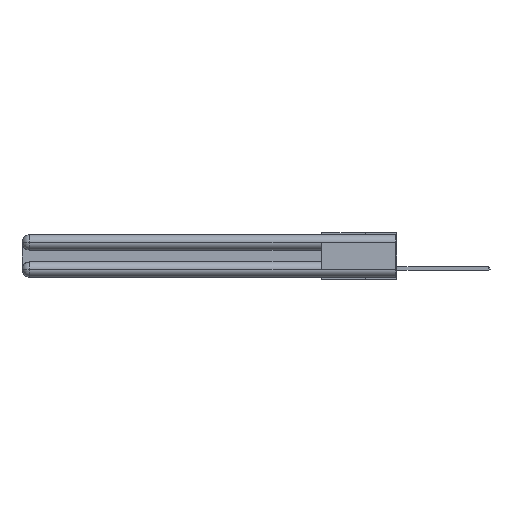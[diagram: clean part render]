
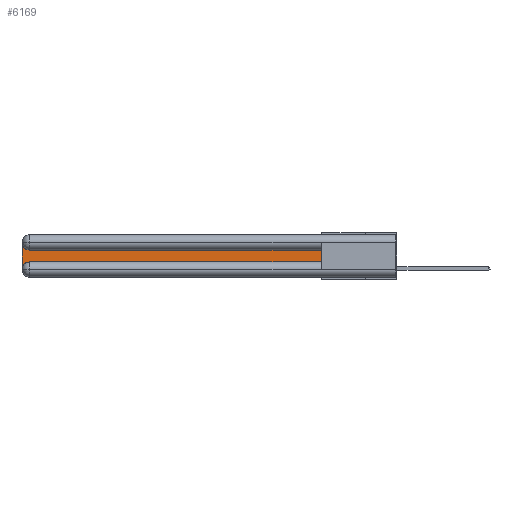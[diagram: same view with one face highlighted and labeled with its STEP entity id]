
A CAD part, left-side view. The second image highlights one B-rep face of the part: STEP entity #6169.
In plain terms, the highlighted planar face has unit normal (-1, 0, 0).
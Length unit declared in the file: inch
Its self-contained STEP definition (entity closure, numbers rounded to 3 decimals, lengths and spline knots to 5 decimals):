
#395 = DIRECTION ( 'NONE',  ( 0., -1., 0. ) ) ;
#704 = VERTEX_POINT ( 'NONE', #10089 ) ;
#2529 = ORIENTED_EDGE ( 'NONE', *, *, #26512, .T. ) ;
#2551 = CARTESIAN_POINT ( 'NONE',  ( 0.075, 2.94, -0.0625 ) ) ;
#2693 = ORIENTED_EDGE ( 'NONE', *, *, #11788, .T. ) ;
#3070 = CARTESIAN_POINT ( 'NONE',  ( 0.075, 3., -0.0625 ) ) ;
#3834 = CARTESIAN_POINT ( 'NONE',  ( 0.075, 2.94, -0.2775 ) ) ;
#5436 = ORIENTED_EDGE ( 'NONE', *, *, #26679, .T. ) ;
#5887 = DIRECTION ( 'NONE',  ( 1., 0., 0. ) ) ;
#6169 = ADVANCED_FACE ( 'NONE', ( #20670 ), #20953, .F. ) ;
#6573 = LINE ( 'NONE', #13060, #21258 ) ;
#6586 = ORIENTED_EDGE ( 'NONE', *, *, #11910, .T. ) ;
#7277 = DIRECTION ( 'NONE',  ( 0., 0., -1. ) ) ;
#7910 = CIRCLE ( 'NONE', #12786, 0.06 ) ;
#7993 = CARTESIAN_POINT ( 'NONE',  ( 0.075, 0.6, -0.2175 ) ) ;
#8329 = VERTEX_POINT ( 'NONE', #24337 ) ;
#9849 = AXIS2_PLACEMENT_3D ( 'NONE', #21363, #16585, #28804 ) ;
#10089 = CARTESIAN_POINT ( 'NONE',  ( 0.075, 0.6, -0.1225 ) ) ;
#10375 = CARTESIAN_POINT ( 'NONE',  ( 0.075, 3., -0.2775 ) ) ;
#11788 = EDGE_CURVE ( 'NONE', #22066, #704, #6573, .T. ) ;
#11910 = EDGE_CURVE ( 'NONE', #704, #8329, #26477, .T. ) ;
#12786 = AXIS2_PLACEMENT_3D ( 'NONE', #2551, #24710, #20321 ) ;
#13060 = CARTESIAN_POINT ( 'NONE',  ( 0.075, 0.6, -0.2175 ) ) ;
#14598 = VECTOR ( 'NONE', #24928, 39.37008 ) ;
#14994 = LINE ( 'NONE', #19904, #19874 ) ;
#15702 = CARTESIAN_POINT ( 'NONE',  ( 0.075, 2.94, -0.2175 ) ) ;
#16585 = DIRECTION ( 'NONE',  ( 1., 0., 0. ) ) ;
#16962 = ORIENTED_EDGE ( 'NONE', *, *, #27528, .T. ) ;
#17598 = ORIENTED_EDGE ( 'NONE', *, *, #28688, .T. ) ;
#18393 = CARTESIAN_POINT ( 'NONE',  ( 0.075, 3., -0.2175 ) ) ;
#18970 = AXIS2_PLACEMENT_3D ( 'NONE', #3834, #5887, #26029 ) ;
#19874 = VECTOR ( 'NONE', #395, 39.37008 ) ;
#19904 = CARTESIAN_POINT ( 'NONE',  ( 0.075, 0.6, -0.2175 ) ) ;
#20286 = CIRCLE ( 'NONE', #18970, 0.06 ) ;
#20321 = DIRECTION ( 'NONE',  ( 0., 0., -1. ) ) ;
#20486 = VERTEX_POINT ( 'NONE', #15702 ) ;
#20670 = FACE_OUTER_BOUND ( 'NONE', #24017, .T. ) ;
#20953 = PLANE ( 'NONE',  #9849 ) ;
#21258 = VECTOR ( 'NONE', #24358, 39.37008 ) ;
#21363 = CARTESIAN_POINT ( 'NONE',  ( 0.075, 3., -0.1225 ) ) ;
#22066 = VERTEX_POINT ( 'NONE', #7993 ) ;
#22728 = VECTOR ( 'NONE', #7277, 39.37008 ) ;
#24017 = EDGE_LOOP ( 'NONE', ( #6586, #17598, #2529, #5436, #16962, #2693 ) ) ;
#24112 = LINE ( 'NONE', #18393, #22728 ) ;
#24337 = CARTESIAN_POINT ( 'NONE',  ( 0.075, 2.94, -0.1225 ) ) ;
#24358 = DIRECTION ( 'NONE',  ( 0., 0., 1. ) ) ;
#24461 = VERTEX_POINT ( 'NONE', #3070 ) ;
#24654 = CARTESIAN_POINT ( 'NONE',  ( 0.075, 0.6, -0.1225 ) ) ;
#24675 = VERTEX_POINT ( 'NONE', #10375 ) ;
#24710 = DIRECTION ( 'NONE',  ( 1., 0., 0. ) ) ;
#24928 = DIRECTION ( 'NONE',  ( 0., 1., 0. ) ) ;
#26029 = DIRECTION ( 'NONE',  ( 0., 0., -1. ) ) ;
#26477 = LINE ( 'NONE', #24654, #14598 ) ;
#26512 = EDGE_CURVE ( 'NONE', #24461, #24675, #24112, .T. ) ;
#26679 = EDGE_CURVE ( 'NONE', #24675, #20486, #20286, .T. ) ;
#27528 = EDGE_CURVE ( 'NONE', #20486, #22066, #14994, .T. ) ;
#28688 = EDGE_CURVE ( 'NONE', #8329, #24461, #7910, .T. ) ;
#28804 = DIRECTION ( 'NONE',  ( 0., 0., -1. ) ) ;
